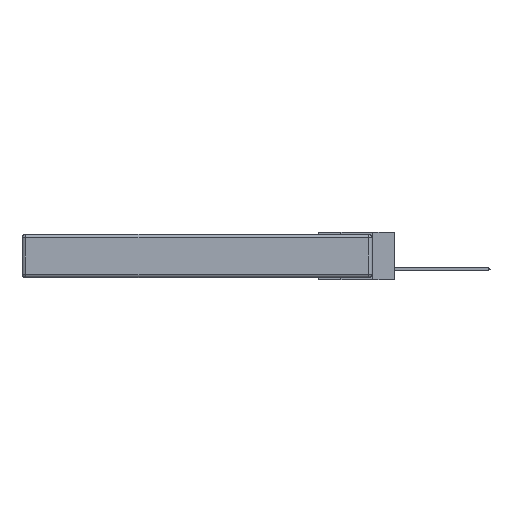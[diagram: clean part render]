
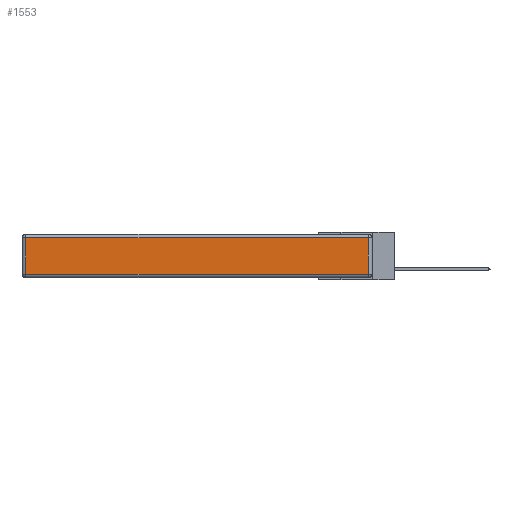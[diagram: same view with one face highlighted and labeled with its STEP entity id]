
A CAD part, left-side view. The second image highlights one B-rep face of the part: STEP entity #1553.
In plain terms, the highlighted planar face has unit normal (-1, 0, 0).
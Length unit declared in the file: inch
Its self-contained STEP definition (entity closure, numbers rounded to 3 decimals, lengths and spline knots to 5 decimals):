
#1553 = ADVANCED_FACE ( 'NONE', ( #13592 ), #6820, .T. ) ;
#2116 = AXIS2_PLACEMENT_3D ( 'NONE', #6748, #19317, #22724 ) ;
#2253 = CARTESIAN_POINT ( 'NONE',  ( 0., 2.72, -0.313 ) ) ;
#3203 = CARTESIAN_POINT ( 'NONE',  ( 0., 2.72, -0.343 ) ) ;
#4942 = DIRECTION ( 'NONE',  ( 0., 0., -1. ) ) ;
#5448 = ORIENTED_EDGE ( 'NONE', *, *, #12103, .T. ) ;
#5896 = VECTOR ( 'NONE', #16580, 39.37008 ) ;
#6469 = CARTESIAN_POINT ( 'NONE',  ( 0., 2.75, -0.03 ) ) ;
#6748 = CARTESIAN_POINT ( 'NONE',  ( 0., 0., -0.343 ) ) ;
#6820 = PLANE ( 'NONE',  #2116 ) ;
#7498 = EDGE_CURVE ( 'NONE', #16377, #22019, #12037, .T. ) ;
#7634 = DIRECTION ( 'NONE',  ( 0., 0., 1. ) ) ;
#7797 = EDGE_LOOP ( 'NONE', ( #18900, #5448, #13171, #20972 ) ) ;
#9659 = CARTESIAN_POINT ( 'NONE',  ( 0., 0.03, -0.343 ) ) ;
#10333 = CARTESIAN_POINT ( 'NONE',  ( 0., 0.03, -0.03 ) ) ;
#10353 = VECTOR ( 'NONE', #4942, 39.37008 ) ;
#10612 = LINE ( 'NONE', #12829, #5896 ) ;
#12037 = LINE ( 'NONE', #3203, #10353 ) ;
#12103 = EDGE_CURVE ( 'NONE', #19823, #22067, #17029, .T. ) ;
#12717 = LINE ( 'NONE', #6469, #22414 ) ;
#12829 = CARTESIAN_POINT ( 'NONE',  ( 0., 0., -0.313 ) ) ;
#13171 = ORIENTED_EDGE ( 'NONE', *, *, #16312, .T. ) ;
#13475 = DIRECTION ( 'NONE',  ( 0., 1., 0. ) ) ;
#13592 = FACE_OUTER_BOUND ( 'NONE', #7797, .T. ) ;
#13620 = EDGE_CURVE ( 'NONE', #22019, #19823, #10612, .T. ) ;
#14155 = CARTESIAN_POINT ( 'NONE',  ( 0., 0.03, -0.313 ) ) ;
#16312 = EDGE_CURVE ( 'NONE', #22067, #16377, #12717, .T. ) ;
#16377 = VERTEX_POINT ( 'NONE', #17626 ) ;
#16472 = VECTOR ( 'NONE', #7634, 39.37008 ) ;
#16580 = DIRECTION ( 'NONE',  ( 0., -1., 0. ) ) ;
#17029 = LINE ( 'NONE', #9659, #16472 ) ;
#17626 = CARTESIAN_POINT ( 'NONE',  ( 0., 2.72, -0.03 ) ) ;
#18900 = ORIENTED_EDGE ( 'NONE', *, *, #13620, .T. ) ;
#19317 = DIRECTION ( 'NONE',  ( -1., 0., 0. ) ) ;
#19823 = VERTEX_POINT ( 'NONE', #14155 ) ;
#20972 = ORIENTED_EDGE ( 'NONE', *, *, #7498, .T. ) ;
#22019 = VERTEX_POINT ( 'NONE', #2253 ) ;
#22067 = VERTEX_POINT ( 'NONE', #10333 ) ;
#22414 = VECTOR ( 'NONE', #13475, 39.37008 ) ;
#22724 = DIRECTION ( 'NONE',  ( 0., 0., 1. ) ) ;
